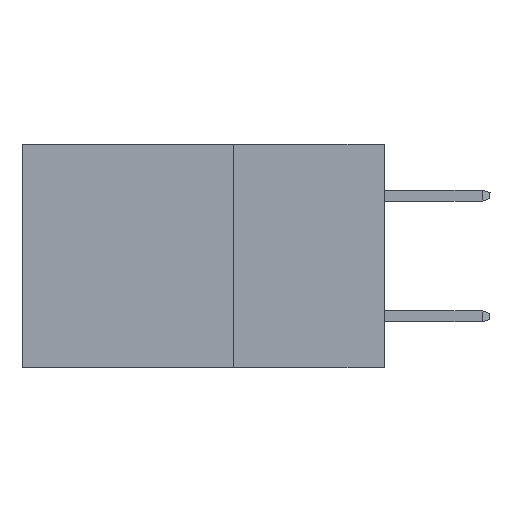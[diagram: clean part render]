
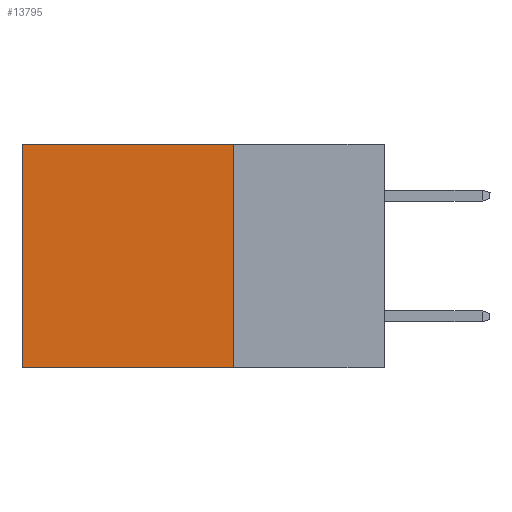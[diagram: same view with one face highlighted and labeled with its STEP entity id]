
A CAD part, left-side view. The second image highlights one B-rep face of the part: STEP entity #13795.
In plain terms, the highlighted planar face has unit normal (-1, 0, 0).
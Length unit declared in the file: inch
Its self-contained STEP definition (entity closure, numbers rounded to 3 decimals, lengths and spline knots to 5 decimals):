
#1262 = LINE ( 'NONE', #13303, #13594 ) ;
#1588 = EDGE_LOOP ( 'NONE', ( #9667, #14411, #14926, #6798 ) ) ;
#1910 = DIRECTION ( 'NONE',  ( 1., 0., 0. ) ) ;
#2075 = CARTESIAN_POINT ( 'NONE',  ( 0.298, 0.6, 0. ) ) ;
#2942 = CARTESIAN_POINT ( 'NONE',  ( 0.298, 0.25, 0. ) ) ;
#3135 = VECTOR ( 'NONE', #16959, 39.37008 ) ;
#5047 = CARTESIAN_POINT ( 'NONE',  ( 0.298, 0.25, -0.37 ) ) ;
#5111 = VERTEX_POINT ( 'NONE', #2075 ) ;
#5360 = LINE ( 'NONE', #14240, #13564 ) ;
#5437 = VERTEX_POINT ( 'NONE', #12201 ) ;
#6264 = EDGE_CURVE ( 'NONE', #13022, #5111, #5360, .T. ) ;
#6388 = LINE ( 'NONE', #6935, #13171 ) ;
#6798 = ORIENTED_EDGE ( 'NONE', *, *, #6264, .T. ) ;
#6935 = CARTESIAN_POINT ( 'NONE',  ( 0.298, 0.25, 0. ) ) ;
#7176 = DIRECTION ( 'NONE',  ( 0., 0., -1. ) ) ;
#7238 = CARTESIAN_POINT ( 'NONE',  ( 0.298, 0.25, 0. ) ) ;
#7274 = FACE_OUTER_BOUND ( 'NONE', #1588, .T. ) ;
#8141 = DIRECTION ( 'NONE',  ( 0., 0., -1. ) ) ;
#9667 = ORIENTED_EDGE ( 'NONE', *, *, #10420, .T. ) ;
#10420 = EDGE_CURVE ( 'NONE', #5111, #16357, #1262, .T. ) ;
#12064 = DIRECTION ( 'NONE',  ( 0., 0., -1. ) ) ;
#12201 = CARTESIAN_POINT ( 'NONE',  ( 0.298, 0.25, -0.37 ) ) ;
#13022 = VERTEX_POINT ( 'NONE', #2942 ) ;
#13171 = VECTOR ( 'NONE', #8141, 39.37008 ) ;
#13303 = CARTESIAN_POINT ( 'NONE',  ( 0.298, 0.6, 0. ) ) ;
#13564 = VECTOR ( 'NONE', #16080, 39.37008 ) ;
#13594 = VECTOR ( 'NONE', #12064, 39.37008 ) ;
#13795 = ADVANCED_FACE ( 'NONE', ( #7274 ), #15047, .F. ) ;
#13826 = LINE ( 'NONE', #5047, #3135 ) ;
#14240 = CARTESIAN_POINT ( 'NONE',  ( 0.298, 0.25, 0. ) ) ;
#14411 = ORIENTED_EDGE ( 'NONE', *, *, #14870, .F. ) ;
#14792 = CARTESIAN_POINT ( 'NONE',  ( 0.298, 0.6, -0.37 ) ) ;
#14870 = EDGE_CURVE ( 'NONE', #5437, #16357, #13826, .T. ) ;
#14926 = ORIENTED_EDGE ( 'NONE', *, *, #16352, .F. ) ;
#15047 = PLANE ( 'NONE',  #15204 ) ;
#15204 = AXIS2_PLACEMENT_3D ( 'NONE', #7238, #1910, #7176 ) ;
#16080 = DIRECTION ( 'NONE',  ( 0., 1., 0. ) ) ;
#16352 = EDGE_CURVE ( 'NONE', #13022, #5437, #6388, .T. ) ;
#16357 = VERTEX_POINT ( 'NONE', #14792 ) ;
#16959 = DIRECTION ( 'NONE',  ( 0., 1., 0. ) ) ;
